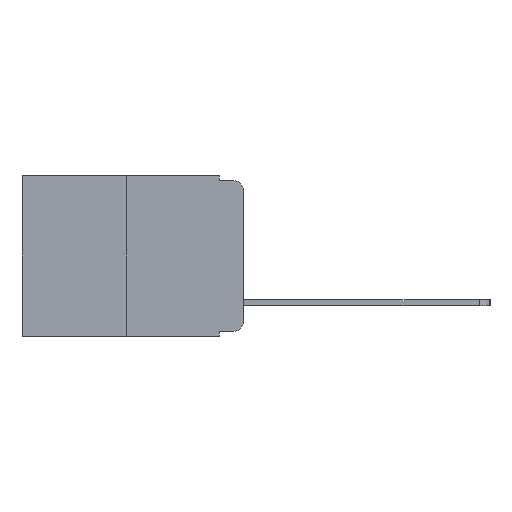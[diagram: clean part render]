
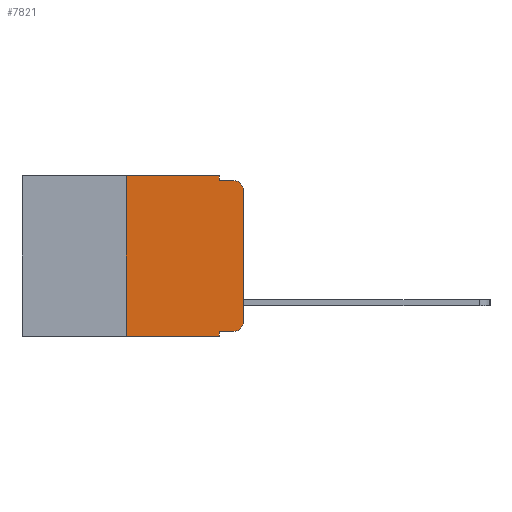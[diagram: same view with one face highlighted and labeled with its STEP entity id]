
A CAD part, left-side view. The second image highlights one B-rep face of the part: STEP entity #7821.
In plain terms, the highlighted planar face has unit normal (-1, 0, 0).
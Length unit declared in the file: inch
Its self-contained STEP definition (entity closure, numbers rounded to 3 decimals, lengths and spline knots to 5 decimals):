
#74 = CARTESIAN_POINT ( 'NONE',  ( 0., 0.051, -0.01 ) ) ;
#128 = CARTESIAN_POINT ( 'NONE',  ( 0., 0.051, -0.333 ) ) ;
#314 = FACE_OUTER_BOUND ( 'NONE', #6510, .T. ) ;
#547 = DIRECTION ( 'NONE',  ( 1., 0., 0. ) ) ;
#676 = EDGE_CURVE ( 'NONE', #6996, #2219, #1453, .T. ) ;
#1008 = DIRECTION ( 'NONE',  ( 0., -1., 0. ) ) ;
#1117 = VERTEX_POINT ( 'NONE', #11346 ) ;
#1453 = LINE ( 'NONE', #7773, #8405 ) ;
#1460 = CARTESIAN_POINT ( 'NONE',  ( 0., 0.051, -0.333 ) ) ;
#1568 = LINE ( 'NONE', #74, #3462 ) ;
#1597 = EDGE_CURVE ( 'NONE', #4599, #3456, #4357, .T. ) ;
#1835 = LINE ( 'NONE', #7674, #6659 ) ;
#1906 = DIRECTION ( 'NONE',  ( 0., 0., -1. ) ) ;
#2129 = ORIENTED_EDGE ( 'NONE', *, *, #5887, .T. ) ;
#2158 = VECTOR ( 'NONE', #3306, 39.37008 ) ;
#2219 = VERTEX_POINT ( 'NONE', #5604 ) ;
#2267 = DIRECTION ( 'NONE',  ( 0., 0., 1. ) ) ;
#2445 = LINE ( 'NONE', #1460, #2158 ) ;
#2701 = ORIENTED_EDGE ( 'NONE', *, *, #6344, .F. ) ;
#2763 = CARTESIAN_POINT ( 'NONE',  ( 0., 0.02, -0.03 ) ) ;
#2851 = EDGE_CURVE ( 'NONE', #6366, #2219, #8559, .T. ) ;
#3306 = DIRECTION ( 'NONE',  ( 0., -1., 0. ) ) ;
#3416 = VERTEX_POINT ( 'NONE', #3636 ) ;
#3451 = CARTESIAN_POINT ( 'NONE',  ( 0., 0.051, 0. ) ) ;
#3456 = VERTEX_POINT ( 'NONE', #3679 ) ;
#3462 = VECTOR ( 'NONE', #1008, 39.37008 ) ;
#3636 = CARTESIAN_POINT ( 'NONE',  ( 0., 0.02, -0.333 ) ) ;
#3679 = CARTESIAN_POINT ( 'NONE',  ( 0., 0.051, -0.01 ) ) ;
#3710 = DIRECTION ( 'NONE',  ( 0., 0., -1. ) ) ;
#3725 = ORIENTED_EDGE ( 'NONE', *, *, #2851, .F. ) ;
#4016 = ORIENTED_EDGE ( 'NONE', *, *, #1597, .F. ) ;
#4019 = ORIENTED_EDGE ( 'NONE', *, *, #9720, .T. ) ;
#4091 = EDGE_CURVE ( 'NONE', #8332, #1117, #9656, .T. ) ;
#4284 = LINE ( 'NONE', #5610, #8738 ) ;
#4291 = DIRECTION ( 'NONE',  ( -1., 0., 0. ) ) ;
#4357 = LINE ( 'NONE', #5516, #6447 ) ;
#4439 = VERTEX_POINT ( 'NONE', #5037 ) ;
#4599 = VERTEX_POINT ( 'NONE', #3451 ) ;
#4636 = AXIS2_PLACEMENT_3D ( 'NONE', #2763, #9064, #3710 ) ;
#4699 = EDGE_CURVE ( 'NONE', #3456, #1117, #1568, .T. ) ;
#4815 = VECTOR ( 'NONE', #5379, 39.37008 ) ;
#5037 = CARTESIAN_POINT ( 'NONE',  ( 0., 0., -0.313 ) ) ;
#5158 = CARTESIAN_POINT ( 'NONE',  ( 0., 0.25, 0. ) ) ;
#5379 = DIRECTION ( 'NONE',  ( 0., 0., 1. ) ) ;
#5516 = CARTESIAN_POINT ( 'NONE',  ( 0., 0.051, 0. ) ) ;
#5604 = CARTESIAN_POINT ( 'NONE',  ( 0., 0.051, -0.343 ) ) ;
#5610 = CARTESIAN_POINT ( 'NONE',  ( 0., 0.473, 0. ) ) ;
#5692 = DIRECTION ( 'NONE',  ( 0., 0., -1. ) ) ;
#5707 = CARTESIAN_POINT ( 'NONE',  ( 0., 0.25, -0.343 ) ) ;
#5887 = EDGE_CURVE ( 'NONE', #4439, #8332, #1835, .T. ) ;
#6027 = CARTESIAN_POINT ( 'NONE',  ( 0., 0.473, 0. ) ) ;
#6176 = VECTOR ( 'NONE', #1906, 39.37008 ) ;
#6247 = ORIENTED_EDGE ( 'NONE', *, *, #11452, .F. ) ;
#6344 = EDGE_CURVE ( 'NONE', #9218, #4599, #4284, .T. ) ;
#6366 = VERTEX_POINT ( 'NONE', #128 ) ;
#6447 = VECTOR ( 'NONE', #5692, 39.37008 ) ;
#6510 = EDGE_LOOP ( 'NONE', ( #2129, #6785, #7792, #4016, #2701, #6247, #8481, #3725, #7070, #4019 ) ) ;
#6648 = CARTESIAN_POINT ( 'NONE',  ( 0., 0., -0.03 ) ) ;
#6659 = VECTOR ( 'NONE', #2267, 39.37008 ) ;
#6785 = ORIENTED_EDGE ( 'NONE', *, *, #4091, .T. ) ;
#6927 = DIRECTION ( 'NONE',  ( 0., 0., -1. ) ) ;
#6996 = VERTEX_POINT ( 'NONE', #5707 ) ;
#6999 = DIRECTION ( 'NONE',  ( 0., -1., 0. ) ) ;
#7070 = ORIENTED_EDGE ( 'NONE', *, *, #8506, .T. ) ;
#7557 = AXIS2_PLACEMENT_3D ( 'NONE', #6027, #547, #6927 ) ;
#7674 = CARTESIAN_POINT ( 'NONE',  ( 0., 0., 0. ) ) ;
#7773 = CARTESIAN_POINT ( 'NONE',  ( 0., 0.473, -0.343 ) ) ;
#7792 = ORIENTED_EDGE ( 'NONE', *, *, #4699, .F. ) ;
#7821 = ADVANCED_FACE ( 'NONE', ( #314 ), #8680, .F. ) ;
#8332 = VERTEX_POINT ( 'NONE', #6648 ) ;
#8405 = VECTOR ( 'NONE', #6999, 39.37008 ) ;
#8481 = ORIENTED_EDGE ( 'NONE', *, *, #676, .T. ) ;
#8506 = EDGE_CURVE ( 'NONE', #6366, #3416, #2445, .T. ) ;
#8559 = LINE ( 'NONE', #10011, #6176 ) ;
#8680 = PLANE ( 'NONE',  #7557 ) ;
#8738 = VECTOR ( 'NONE', #10929, 39.37008 ) ;
#9064 = DIRECTION ( 'NONE',  ( -1., 0., 0. ) ) ;
#9218 = VERTEX_POINT ( 'NONE', #5158 ) ;
#9646 = CARTESIAN_POINT ( 'NONE',  ( 0., 0.02, -0.313 ) ) ;
#9656 = CIRCLE ( 'NONE', #4636, 0.02 ) ;
#9720 = EDGE_CURVE ( 'NONE', #3416, #4439, #10986, .T. ) ;
#10011 = CARTESIAN_POINT ( 'NONE',  ( 0., 0.051, 0. ) ) ;
#10139 = LINE ( 'NONE', #11498, #4815 ) ;
#10529 = DIRECTION ( 'NONE',  ( 0., 0., -1. ) ) ;
#10929 = DIRECTION ( 'NONE',  ( 0., -1., 0. ) ) ;
#10986 = CIRCLE ( 'NONE', #11568, 0.02 ) ;
#11346 = CARTESIAN_POINT ( 'NONE',  ( 0., 0.02, -0.01 ) ) ;
#11452 = EDGE_CURVE ( 'NONE', #6996, #9218, #10139, .T. ) ;
#11498 = CARTESIAN_POINT ( 'NONE',  ( 0., 0.25, 0. ) ) ;
#11568 = AXIS2_PLACEMENT_3D ( 'NONE', #9646, #4291, #10529 ) ;
